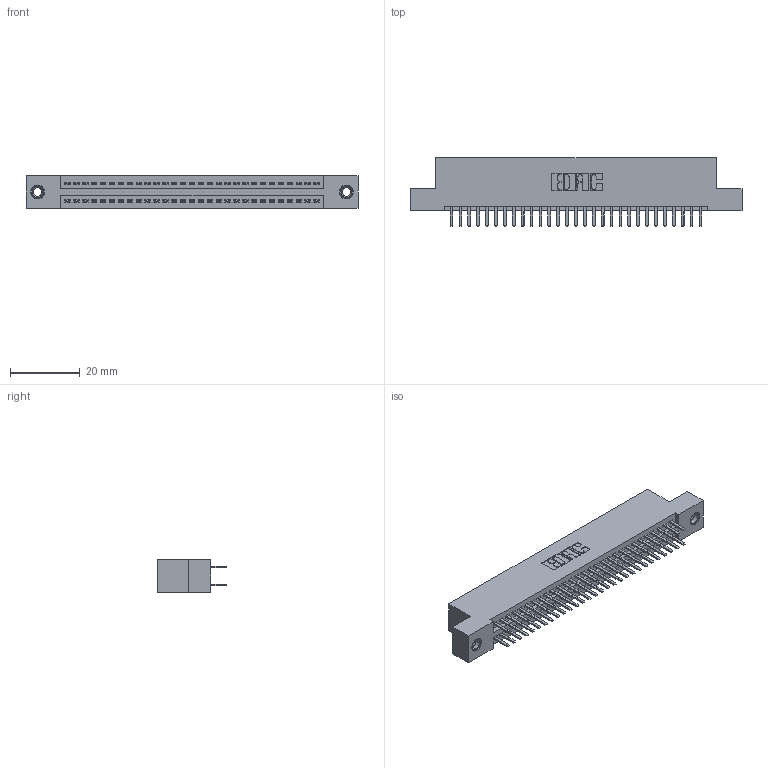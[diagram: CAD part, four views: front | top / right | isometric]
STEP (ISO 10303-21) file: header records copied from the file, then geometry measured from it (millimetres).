
FILE_DESCRIPTION (( 'STEP AP203' ), '1' );
FILE_NAME ('345-058-520-207.STEP', '2018-09-19T04:43:20', ( '' ), ( '' ), 'SwSTEP 2.0', 'SolidWorks 2016', '' );
FILE_SCHEMA (( 'CONFIG_CONTROL_DESIGN' ));
Length unit declared in the file: inch
Products named in the file (4): 345-058-520-207; 345 Part_Flush Mounting Lugs - 0.156 Dia-TI; 345-292-001_345-293-120; 345-250-001_345-250-005-103
Assembly tree (61 placements, depth 2):
  345-058-520-207
    345 Part_Flush Mounting Lugs - 0.156 Dia-TI
    345-292-001_345-293-120  x58
    345-250-001_345-250-005-103  x2
Bounding box: 94.87 x 19.68 x 9.4 mm (x, y, z)
Volume: 589.8 mm3; surface area: 13101.7 mm2
Topology: 60 solids, 61 shells, 3318 faces, 9583 edges, 6226 vertices
Faces by surface type: plane 2142, cylinder 1160, cone 12, torus 4
Entity records: 25804 total; most frequent: CARTESIAN_POINT 4331, ORIENTED_EDGE 4246, DIRECTION 3849, EDGE_CURVE 2123, LINE 1851, VECTOR 1851, VERTEX_POINT 1408, AXIS2_PLACEMENT_3D 999
